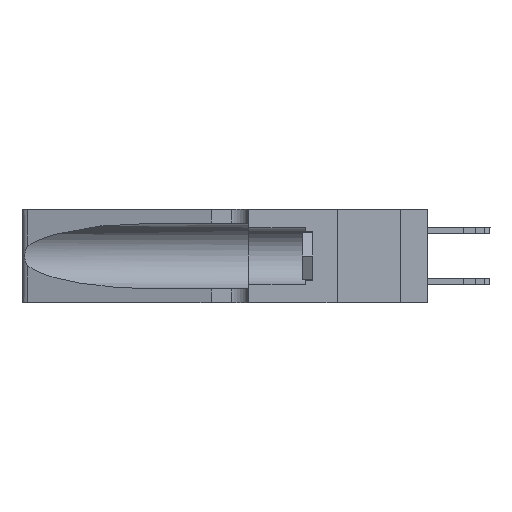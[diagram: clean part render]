
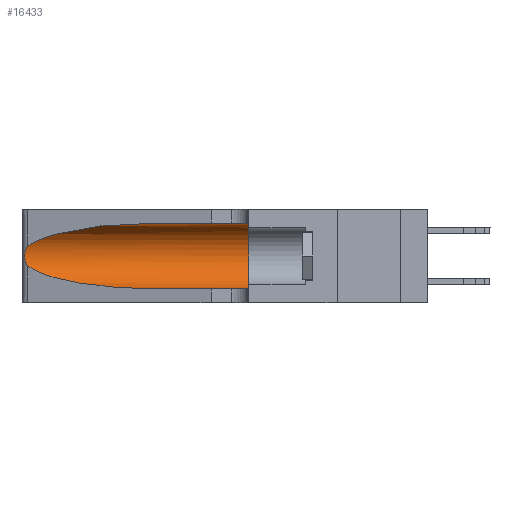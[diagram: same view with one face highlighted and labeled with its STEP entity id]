
A CAD part, left-side view. The second image highlights one B-rep face of the part: STEP entity #16433.
In plain terms, the highlighted cylindrical face has radius 3.308 mm (diameter 6.617 mm), a partial arc.
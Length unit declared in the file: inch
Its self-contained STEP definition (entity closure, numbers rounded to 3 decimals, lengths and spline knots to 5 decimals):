
#481 = VERTEX_POINT ( 'NONE', #8709 ) ;
#1414 = ORIENTED_EDGE ( 'NONE', *, *, #4972, .T. ) ;
#1562 = ORIENTED_EDGE ( 'NONE', *, *, #15373, .F. ) ;
#1621 = CARTESIAN_POINT ( 'NONE',  ( 0.25487, 1.22718, 0.14631 ) ) ;
#2223 = VERTEX_POINT ( 'NONE', #8364 ) ;
#2256 = CARTESIAN_POINT ( 'NONE',  ( 0.1305, 0.72297, 0.31525 ) ) ;
#2763 = DIRECTION ( 'NONE',  ( 0., -1., 0. ) ) ;
#3466 = CARTESIAN_POINT ( 'NONE',  ( 0.25854, 1.2359, 0.20912 ) ) ;
#3637 = CARTESIAN_POINT ( 'NONE',  ( 0.26017, 1.23833, 0.17102 ) ) ;
#4418 = LINE ( 'NONE', #9689, #6641 ) ;
#4656 = ORIENTED_EDGE ( 'NONE', *, *, #5504, .T. ) ;
#4712 = CARTESIAN_POINT ( 'NONE',  ( 0.18966, 0.96281, 0.31525 ) ) ;
#4972 = EDGE_CURVE ( 'NONE', #10860, #481, #8448, .T. ) ;
#5179 = CARTESIAN_POINT ( 'NONE',  ( 0.1305, 0.72297, 0.05475 ) ) ;
#5449 = DIRECTION ( 'NONE',  ( 0., 1., 0. ) ) ;
#5504 = EDGE_CURVE ( 'NONE', #9190, #10860, #20997, .T. ) ;
#6409 = ORIENTED_EDGE ( 'NONE', *, *, #17805, .T. ) ;
#6641 = VECTOR ( 'NONE', #12212, 39.37008 ) ;
#7268 = CIRCLE ( 'NONE', #16197, 0.13025 ) ;
#7381 = CARTESIAN_POINT ( 'NONE',  ( 0.2373, 1.15595, 0.08982 ) ) ;
#7429 = CARTESIAN_POINT ( 'NONE',  ( 0.25487, 1.22718, 0.22369 ) ) ;
#8333 = VERTEX_POINT ( 'NONE', #17781 ) ;
#8364 = CARTESIAN_POINT ( 'NONE',  ( 0.1305, 0.72297, 0.31525 ) ) ;
#8448 = LINE ( 'NONE', #11025, #9739 ) ;
#8625 = ORIENTED_EDGE ( 'NONE', *, *, #15473, .F. ) ;
#8709 = CARTESIAN_POINT ( 'NONE',  ( 0.1305, 0.35, 0.05475 ) ) ;
#8797 = FACE_OUTER_BOUND ( 'NONE', #8901, .T. ) ;
#8901 = EDGE_LOOP ( 'NONE', ( #9419, #6409, #4656, #1414, #1562, #8625 ) ) ;
#9190 = VERTEX_POINT ( 'NONE', #25179 ) ;
#9419 = ORIENTED_EDGE ( 'NONE', *, *, #15764, .T. ) ;
#9554 = CARTESIAN_POINT ( 'NONE',  ( 0.26075, 1.23896, 0.178 ) ) ;
#9689 = CARTESIAN_POINT ( 'NONE',  ( 0.1305, 1.61858, 0.31525 ) ) ;
#9739 = VECTOR ( 'NONE', #15390, 39.37008 ) ;
#10659 =( BOUNDED_CURVE ( )  B_SPLINE_CURVE ( 3, ( #2256, #4712, #15074, #18772 ),
 .UNSPECIFIED., .F., .T. ) 
 B_SPLINE_CURVE_WITH_KNOTS ( ( 4, 4 ),
 ( 1.5708, 2.84003 ),
 .UNSPECIFIED. ) 
 CURVE ( )  GEOMETRIC_REPRESENTATION_ITEM ( )  RATIONAL_B_SPLINE_CURVE ( ( 1., 0.87, 0.87, 1. ) ) 
 REPRESENTATION_ITEM ( '' )  );
#10860 = VERTEX_POINT ( 'NONE', #13746 ) ;
#11025 = CARTESIAN_POINT ( 'NONE',  ( 0.1305, 1.61858, 0.05475 ) ) ;
#11564 = CARTESIAN_POINT ( 'NONE',  ( 0.25789, 1.23486, 0.15765 ) ) ;
#12212 = DIRECTION ( 'NONE',  ( 0., -1., 0. ) ) ;
#13589 = CARTESIAN_POINT ( 'NONE',  ( 0.25639, 1.23186, 0.15144 ) ) ;
#13679 = CARTESIAN_POINT ( 'NONE',  ( 0.25555, 1.22994, 0.2215 ) ) ;
#13746 = CARTESIAN_POINT ( 'NONE',  ( 0.1305, 0.72297, 0.05475 ) ) ;
#15074 = CARTESIAN_POINT ( 'NONE',  ( 0.2373, 1.15595, 0.28018 ) ) ;
#15373 = EDGE_CURVE ( 'NONE', #8333, #481, #7268, .T. ) ;
#15390 = DIRECTION ( 'NONE',  ( 0., -1., 0. ) ) ;
#15473 = EDGE_CURVE ( 'NONE', #2223, #8333, #4418, .T. ) ;
#15764 = EDGE_CURVE ( 'NONE', #2223, #25933, #10659, .T. ) ;
#16197 = AXIS2_PLACEMENT_3D ( 'NONE', #17475, #5449, #17825 ) ;
#16433 = ADVANCED_FACE ( 'NONE', ( #8797 ), #24212, .F. ) ;
#17475 = CARTESIAN_POINT ( 'NONE',  ( 0.1305, 0.35, 0.185 ) ) ;
#17596 = CARTESIAN_POINT ( 'NONE',  ( 0.25555, 1.22993, 0.14849 ) ) ;
#17688 = CARTESIAN_POINT ( 'NONE',  ( 0.25639, 1.23184, 0.21858 ) ) ;
#17781 = CARTESIAN_POINT ( 'NONE',  ( 0.1305, 0.35, 0.31525 ) ) ;
#17805 = EDGE_CURVE ( 'NONE', #25933, #9190, #22746, .T. ) ;
#17825 = DIRECTION ( 'NONE',  ( 0., 0., 1. ) ) ;
#18380 = DIRECTION ( 'NONE',  ( 0., 0., -1. ) ) ;
#18772 = CARTESIAN_POINT ( 'NONE',  ( 0.25487, 1.22718, 0.22369 ) ) ;
#19418 = CARTESIAN_POINT ( 'NONE',  ( 0.25487, 1.22718, 0.14631 ) ) ;
#19546 = CARTESIAN_POINT ( 'NONE',  ( 0.26018, 1.23835, 0.19895 ) ) ;
#20615 = CARTESIAN_POINT ( 'NONE',  ( 0.25487, 1.22718, 0.22369 ) ) ;
#20997 =( BOUNDED_CURVE ( )  B_SPLINE_CURVE ( 3, ( #19418, #7381, #23210, #5179 ),
 .UNSPECIFIED., .F., .F. ) 
 B_SPLINE_CURVE_WITH_KNOTS ( ( 4, 4 ),
 ( 3.44316, 4.71239 ),
 .UNSPECIFIED. ) 
 CURVE ( )  GEOMETRIC_REPRESENTATION_ITEM ( )  RATIONAL_B_SPLINE_CURVE ( ( 1., 0.87, 0.87, 1. ) ) 
 REPRESENTATION_ITEM ( '' )  );
#21562 = CARTESIAN_POINT ( 'NONE',  ( 0.26075, 1.23896, 0.19203 ) ) ;
#22719 = CARTESIAN_POINT ( 'NONE',  ( 0.1305, 1.61858, 0.185 ) ) ;
#22746 = B_SPLINE_CURVE_WITH_KNOTS ( 'NONE', 3,
 ( #7429, #13679, #17688, #25670, #3466, #19546, #21562, #9554, #3637, #23613, #11564, #13589, #17596, #1621 ),
 .UNSPECIFIED., .F., .F.,
 ( 4, 2, 2, 2, 2, 2, 4 ),
 ( 0., 0.00027, 0.00053, 0.00107, 0.0016, 0.00187, 0.00214 ),
 .UNSPECIFIED. ) ;
#23210 = CARTESIAN_POINT ( 'NONE',  ( 0.18966, 0.96281, 0.05475 ) ) ;
#23613 = CARTESIAN_POINT ( 'NONE',  ( 0.25856, 1.23593, 0.16098 ) ) ;
#24207 = AXIS2_PLACEMENT_3D ( 'NONE', #22719, #2763, #18380 ) ;
#24212 = CYLINDRICAL_SURFACE ( 'NONE', #24207, 0.13025 ) ;
#25179 = CARTESIAN_POINT ( 'NONE',  ( 0.25487, 1.22718, 0.14631 ) ) ;
#25670 = CARTESIAN_POINT ( 'NONE',  ( 0.25787, 1.23484, 0.2124 ) ) ;
#25933 = VERTEX_POINT ( 'NONE', #20615 ) ;
